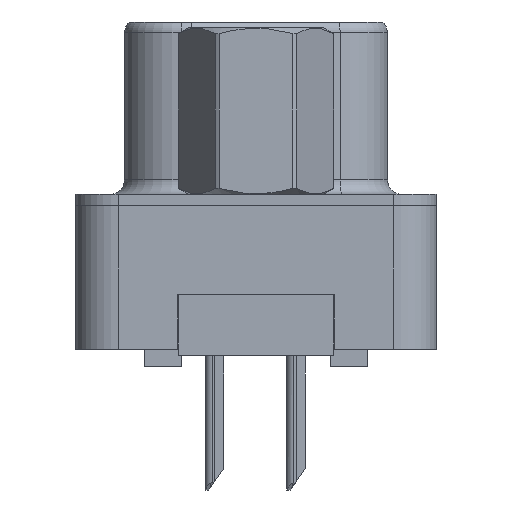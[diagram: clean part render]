
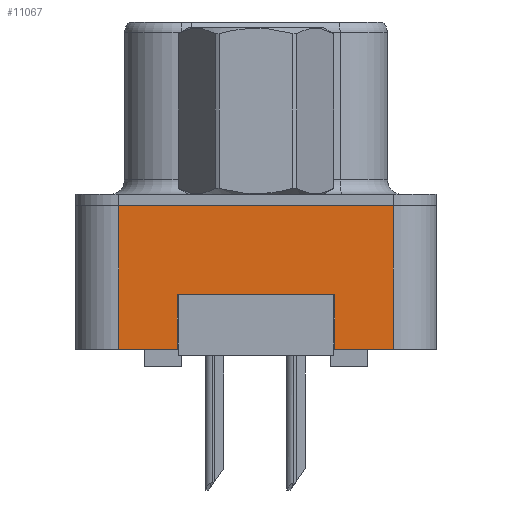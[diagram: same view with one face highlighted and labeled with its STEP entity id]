
A CAD part, left-side view. The second image highlights one B-rep face of the part: STEP entity #11067.
In plain terms, the highlighted planar face has unit normal (-1, 0, 0).
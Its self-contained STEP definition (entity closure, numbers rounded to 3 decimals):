
#678 = EDGE_CURVE ( 'NONE', #31510, #22649, #10477, .T. ) ;
#817 = CARTESIAN_POINT ( 'NONE',  ( -2.91, -4.775, -5. ) ) ;
#1238 = DIRECTION ( 'NONE',  ( 0., 0., 1. ) ) ;
#1613 = CARTESIAN_POINT ( 'NONE',  ( -2.91, 2.75, -3.1 ) ) ;
#2696 = CARTESIAN_POINT ( 'NONE',  ( -2.91, -4.775, -5. ) ) ;
#3659 = CARTESIAN_POINT ( 'NONE',  ( -2.91, -4.775, -5. ) ) ;
#3683 = DIRECTION ( 'NONE',  ( 0., -1., 0. ) ) ;
#3739 = VECTOR ( 'NONE', #18167, 1000. ) ;
#4836 = ORIENTED_EDGE ( 'NONE', *, *, #13197, .F. ) ;
#4913 = LINE ( 'NONE', #15426, #3739 ) ;
#5320 = CARTESIAN_POINT ( 'NONE',  ( -2.91, 4.775, -5. ) ) ;
#5914 = LINE ( 'NONE', #18664, #28710 ) ;
#6394 = VERTEX_POINT ( 'NONE', #23820 ) ;
#7128 = CARTESIAN_POINT ( 'NONE',  ( -2.91, -4.775, -5. ) ) ;
#7468 = VECTOR ( 'NONE', #21334, 1000. ) ;
#7469 = AXIS2_PLACEMENT_3D ( 'NONE', #2696, #8194, #10777 ) ;
#7633 = DIRECTION ( 'NONE',  ( 0., 0., -1. ) ) ;
#7708 = ORIENTED_EDGE ( 'NONE', *, *, #24145, .T. ) ;
#8194 = DIRECTION ( 'NONE',  ( -1., 0., 0. ) ) ;
#8982 = LINE ( 'NONE', #3659, #15171 ) ;
#9183 = LINE ( 'NONE', #1613, #23106 ) ;
#10477 = LINE ( 'NONE', #5320, #7468 ) ;
#10777 = DIRECTION ( 'NONE',  ( 0., 0., 1. ) ) ;
#11067 = ADVANCED_FACE ( 'NONE', ( #13702 ), #13016, .T. ) ;
#11068 = ORIENTED_EDGE ( 'NONE', *, *, #32739, .T. ) ;
#12896 = EDGE_LOOP ( 'NONE', ( #24721, #7708, #19183, #4836, #29206, #11068, #26940, #25790 ) ) ;
#13016 = PLANE ( 'NONE',  #7469 ) ;
#13197 = EDGE_CURVE ( 'NONE', #22649, #17458, #4913, .T. ) ;
#13702 = FACE_OUTER_BOUND ( 'NONE', #12896, .T. ) ;
#15171 = VECTOR ( 'NONE', #1238, 1000. ) ;
#15426 = CARTESIAN_POINT ( 'NONE',  ( -2.91, -4.775, 0. ) ) ;
#15974 = CARTESIAN_POINT ( 'NONE',  ( -2.91, -2.75, -3.1 ) ) ;
#16074 = VECTOR ( 'NONE', #7633, 1000. ) ;
#16739 = DIRECTION ( 'NONE',  ( 0., 0., -1. ) ) ;
#17458 = VERTEX_POINT ( 'NONE', #30224 ) ;
#18167 = DIRECTION ( 'NONE',  ( 0., -1., 0. ) ) ;
#18296 = LINE ( 'NONE', #31938, #16074 ) ;
#18664 = CARTESIAN_POINT ( 'NONE',  ( -2.91, 2.75, -3.1 ) ) ;
#19101 = VERTEX_POINT ( 'NONE', #22284 ) ;
#19118 = EDGE_CURVE ( 'NONE', #24196, #24049, #9183, .T. ) ;
#19183 = ORIENTED_EDGE ( 'NONE', *, *, #27543, .T. ) ;
#19345 = CARTESIAN_POINT ( 'NONE',  ( -2.91, -4.775, -5. ) ) ;
#19868 = DIRECTION ( 'NONE',  ( 0., 1., 0. ) ) ;
#21334 = DIRECTION ( 'NONE',  ( 0., 0., 1. ) ) ;
#21609 = VECTOR ( 'NONE', #29105, 1000. ) ;
#22284 = CARTESIAN_POINT ( 'NONE',  ( -2.91, 2.75, -5. ) ) ;
#22594 = EDGE_CURVE ( 'NONE', #24049, #19101, #5914, .T. ) ;
#22649 = VERTEX_POINT ( 'NONE', #26607 ) ;
#23069 = CARTESIAN_POINT ( 'NONE',  ( -2.91, 2.75, -3.1 ) ) ;
#23106 = VECTOR ( 'NONE', #19868, 1000. ) ;
#23483 = VERTEX_POINT ( 'NONE', #7128 ) ;
#23730 = EDGE_CURVE ( 'NONE', #24196, #6394, #18296, .T. ) ;
#23820 = CARTESIAN_POINT ( 'NONE',  ( -2.91, -2.75, -5. ) ) ;
#24049 = VERTEX_POINT ( 'NONE', #23069 ) ;
#24145 = EDGE_CURVE ( 'NONE', #6394, #23483, #24253, .T. ) ;
#24196 = VERTEX_POINT ( 'NONE', #15974 ) ;
#24253 = LINE ( 'NONE', #817, #21609 ) ;
#24721 = ORIENTED_EDGE ( 'NONE', *, *, #23730, .T. ) ;
#25790 = ORIENTED_EDGE ( 'NONE', *, *, #19118, .F. ) ;
#26357 = CARTESIAN_POINT ( 'NONE',  ( -2.91, 4.775, -5. ) ) ;
#26607 = CARTESIAN_POINT ( 'NONE',  ( -2.91, 4.775, 0. ) ) ;
#26940 = ORIENTED_EDGE ( 'NONE', *, *, #22594, .F. ) ;
#27543 = EDGE_CURVE ( 'NONE', #23483, #17458, #8982, .T. ) ;
#27627 = LINE ( 'NONE', #19345, #29859 ) ;
#28710 = VECTOR ( 'NONE', #16739, 1000. ) ;
#29105 = DIRECTION ( 'NONE',  ( 0., -1., 0. ) ) ;
#29206 = ORIENTED_EDGE ( 'NONE', *, *, #678, .F. ) ;
#29859 = VECTOR ( 'NONE', #3683, 1000. ) ;
#30224 = CARTESIAN_POINT ( 'NONE',  ( -2.91, -4.775, 0. ) ) ;
#31510 = VERTEX_POINT ( 'NONE', #26357 ) ;
#31938 = CARTESIAN_POINT ( 'NONE',  ( -2.91, -2.75, -3.1 ) ) ;
#32739 = EDGE_CURVE ( 'NONE', #31510, #19101, #27627, .T. ) ;
